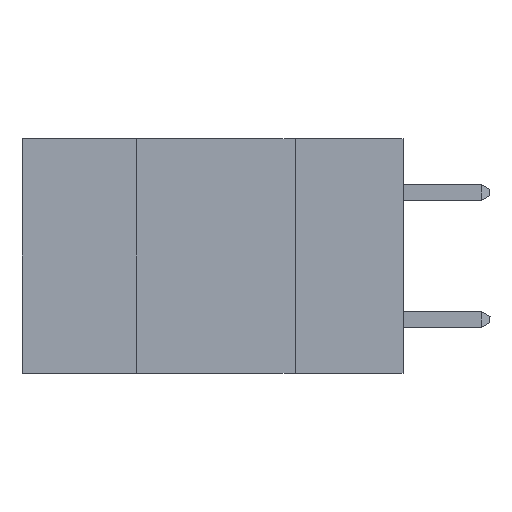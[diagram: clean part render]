
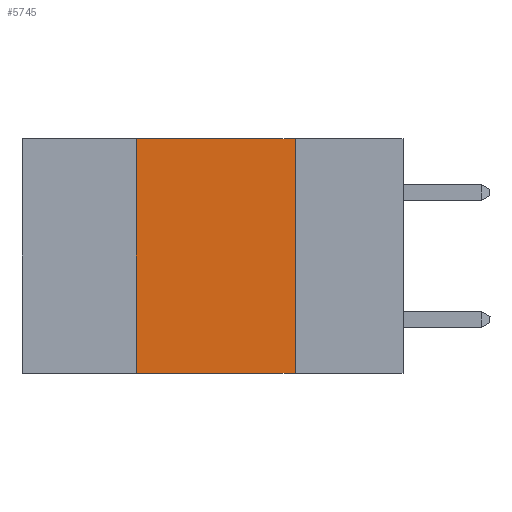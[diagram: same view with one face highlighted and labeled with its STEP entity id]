
A CAD part, left-side view. The second image highlights one B-rep face of the part: STEP entity #5745.
In plain terms, the highlighted planar face has unit normal (-1, 0, 0).
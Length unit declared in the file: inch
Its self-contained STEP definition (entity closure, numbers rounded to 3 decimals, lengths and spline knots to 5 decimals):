
#478 = CARTESIAN_POINT ( 'NONE',  ( 0., 0.17, 0. ) ) ;
#503 = ORIENTED_EDGE ( 'NONE', *, *, #11870, .F. ) ;
#863 = PLANE ( 'NONE',  #9107 ) ;
#1349 = CARTESIAN_POINT ( 'NONE',  ( 0., 0.6, -0.37 ) ) ;
#1569 = LINE ( 'NONE', #7942, #1877 ) ;
#1877 = VECTOR ( 'NONE', #2305, 39.37008 ) ;
#1897 = VERTEX_POINT ( 'NONE', #7380 ) ;
#2305 = DIRECTION ( 'NONE',  ( 0., 0., 1. ) ) ;
#2912 = LINE ( 'NONE', #4804, #6646 ) ;
#3362 = LINE ( 'NONE', #11749, #4606 ) ;
#4606 = VECTOR ( 'NONE', #5977, 39.37008 ) ;
#4804 = CARTESIAN_POINT ( 'NONE',  ( 0., 0.6, 0. ) ) ;
#4852 = VERTEX_POINT ( 'NONE', #11987 ) ;
#4963 = DIRECTION ( 'NONE',  ( 0., -1., 0. ) ) ;
#5505 = EDGE_CURVE ( 'NONE', #4852, #1897, #8578, .T. ) ;
#5519 = ORIENTED_EDGE ( 'NONE', *, *, #6117, .F. ) ;
#5628 = VERTEX_POINT ( 'NONE', #10963 ) ;
#5745 = ADVANCED_FACE ( 'NONE', ( #6417 ), #863, .F. ) ;
#5977 = DIRECTION ( 'NONE',  ( 0., 0., -1. ) ) ;
#6020 = EDGE_CURVE ( 'NONE', #7779, #1897, #3362, .T. ) ;
#6117 = EDGE_CURVE ( 'NONE', #4852, #5628, #1569, .T. ) ;
#6417 = FACE_OUTER_BOUND ( 'NONE', #9546, .T. ) ;
#6646 = VECTOR ( 'NONE', #10435, 39.37008 ) ;
#7380 = CARTESIAN_POINT ( 'NONE',  ( 0., 0.17, -0.37 ) ) ;
#7779 = VERTEX_POINT ( 'NONE', #478 ) ;
#7942 = CARTESIAN_POINT ( 'NONE',  ( 0., 0.42, 0. ) ) ;
#8085 = ORIENTED_EDGE ( 'NONE', *, *, #6020, .F. ) ;
#8578 = LINE ( 'NONE', #1349, #9384 ) ;
#9107 = AXIS2_PLACEMENT_3D ( 'NONE', #9112, #10270, #11072 ) ;
#9112 = CARTESIAN_POINT ( 'NONE',  ( 0., 0.6, 0. ) ) ;
#9125 = ORIENTED_EDGE ( 'NONE', *, *, #5505, .T. ) ;
#9384 = VECTOR ( 'NONE', #4963, 39.37008 ) ;
#9546 = EDGE_LOOP ( 'NONE', ( #8085, #503, #5519, #9125 ) ) ;
#10270 = DIRECTION ( 'NONE',  ( 1., 0., 0. ) ) ;
#10435 = DIRECTION ( 'NONE',  ( 0., -1., 0. ) ) ;
#10963 = CARTESIAN_POINT ( 'NONE',  ( 0., 0.42, 0. ) ) ;
#11072 = DIRECTION ( 'NONE',  ( 0., 0., -1. ) ) ;
#11749 = CARTESIAN_POINT ( 'NONE',  ( 0., 0.17, 0. ) ) ;
#11870 = EDGE_CURVE ( 'NONE', #5628, #7779, #2912, .T. ) ;
#11987 = CARTESIAN_POINT ( 'NONE',  ( 0., 0.42, -0.37 ) ) ;
